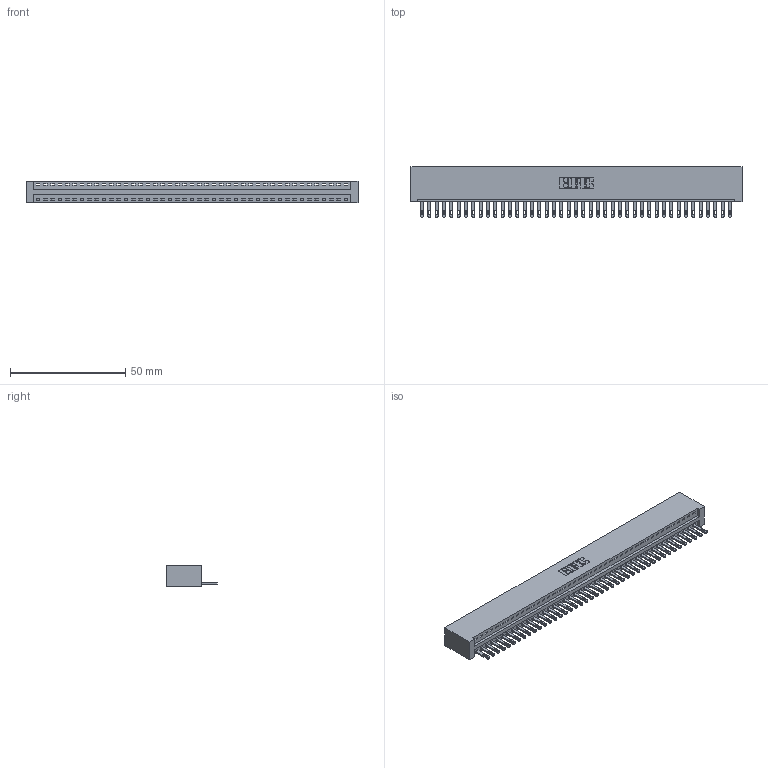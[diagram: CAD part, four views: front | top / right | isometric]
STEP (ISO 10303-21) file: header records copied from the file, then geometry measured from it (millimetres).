
FILE_DESCRIPTION (( 'STEP AP203' ), '1' );
FILE_NAME ('896-043-500-101.STEP', '2021-07-27T21:46:42', ( '' ), ( '' ), 'SwSTEP 2.0', 'SolidWorks 2020', '' );
FILE_SCHEMA (( 'CONFIG_CONTROL_DESIGN' ));
Length unit declared in the file: inch
Products named in the file (3): 345-292-001_345-293-100; 896-043-500-101; 846 Part_No Mounting Lugs
Assembly tree (44 placements, depth 2):
  896-043-500-101
    846 Part_No Mounting Lugs
    345-292-001_345-293-100  x43
Bounding box: 143.76 x 21.84 x 9.4 mm (x, y, z)
Volume: 14344.3 mm3; surface area: 18114.6 mm2
Topology: 44 solids, 44 shells, 2436 faces, 7529 edges, 5018 vertices
Faces by surface type: plane 1534, cylinder 902
Entity records: 26205 total; most frequent: CARTESIAN_POINT 4497, ORIENTED_EDGE 4474, DIRECTION 3963, EDGE_CURVE 2237, LINE 1937, VECTOR 1937, VERTEX_POINT 1490, AXIS2_PLACEMENT_3D 1013
